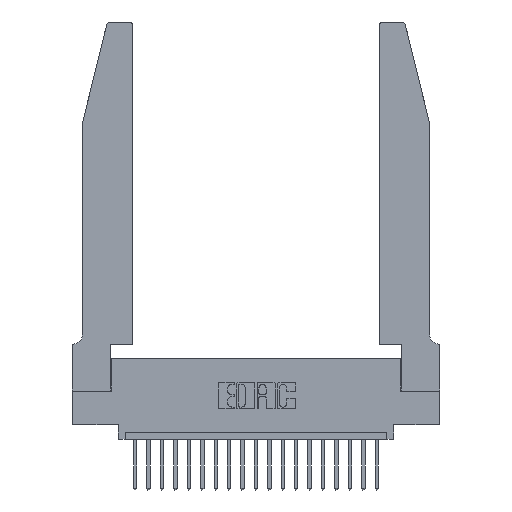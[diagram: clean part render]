
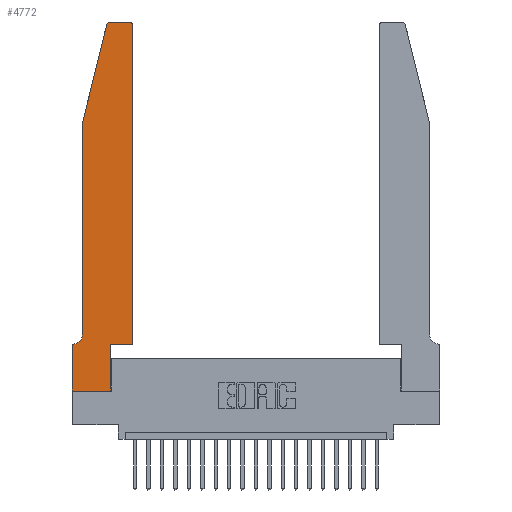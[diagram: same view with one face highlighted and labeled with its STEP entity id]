
A CAD part, top view. The second image highlights one B-rep face of the part: STEP entity #4772.
In plain terms, the highlighted planar face has unit normal (0, 0, 1).
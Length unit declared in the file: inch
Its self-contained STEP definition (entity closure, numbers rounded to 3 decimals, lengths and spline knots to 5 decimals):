
#226 = EDGE_CURVE ( 'NONE', #18353, #14576, #21338, .T. ) ;
#372 = VERTEX_POINT ( 'NONE', #13995 ) ;
#483 = DIRECTION ( 'NONE',  ( 0., 0., 1. ) ) ;
#504 = DIRECTION ( 'NONE',  ( -1., 0., 0. ) ) ;
#871 = VERTEX_POINT ( 'NONE', #3465 ) ;
#1486 = VECTOR ( 'NONE', #11766, 39.37008 ) ;
#1826 = DIRECTION ( 'NONE',  ( 0., -1., 0. ) ) ;
#1968 = ORIENTED_EDGE ( 'NONE', *, *, #3648, .T. ) ;
#2266 = DIRECTION ( 'NONE',  ( 1., 0., 0. ) ) ;
#2371 = EDGE_CURVE ( 'NONE', #14576, #21226, #3385, .T. ) ;
#3284 = DIRECTION ( 'NONE',  ( -1., 0., 0. ) ) ;
#3385 = LINE ( 'NONE', #17024, #1486 ) ;
#3426 = CARTESIAN_POINT ( 'NONE',  ( 0., 0.35, 0.37 ) ) ;
#3465 = CARTESIAN_POINT ( 'NONE',  ( 0.4505, 0.35, 0.37 ) ) ;
#3476 = EDGE_CURVE ( 'NONE', #6200, #7450, #18673, .T. ) ;
#3612 = CIRCLE ( 'NONE', #15629, 0.07 ) ;
#3648 = EDGE_CURVE ( 'NONE', #12119, #12904, #3612, .T. ) ;
#3975 = CARTESIAN_POINT ( 'NONE',  ( 0.0755, 0.42, 0.37 ) ) ;
#4287 = LINE ( 'NONE', #19986, #12368 ) ;
#4311 = VECTOR ( 'NONE', #3284, 39.37008 ) ;
#4448 = VERTEX_POINT ( 'NONE', #13003 ) ;
#4772 = ADVANCED_FACE ( 'NONE', ( #4918 ), #11922, .T. ) ;
#4799 = LINE ( 'NONE', #17687, #5856 ) ;
#4854 = DIRECTION ( 'NONE',  ( 0., 1., 0. ) ) ;
#4918 = FACE_OUTER_BOUND ( 'NONE', #9921, .T. ) ;
#4961 = EDGE_CURVE ( 'NONE', #871, #17091, #15904, .T. ) ;
#5109 = DIRECTION ( 'NONE',  ( 1., 0., 0. ) ) ;
#5128 = ORIENTED_EDGE ( 'NONE', *, *, #3476, .T. ) ;
#5356 = VECTOR ( 'NONE', #1826, 39.37008 ) ;
#5388 = ORIENTED_EDGE ( 'NONE', *, *, #16387, .T. ) ;
#5488 = VERTEX_POINT ( 'NONE', #15908 ) ;
#5856 = VECTOR ( 'NONE', #2266, 39.37008 ) ;
#6200 = VERTEX_POINT ( 'NONE', #21946 ) ;
#6231 = DIRECTION ( 'NONE',  ( -0.239, -0.971, 0. ) ) ;
#6985 = CARTESIAN_POINT ( 'NONE',  ( 0., 0.35, 0.37 ) ) ;
#7149 = EDGE_CURVE ( 'NONE', #5488, #871, #4799, .T. ) ;
#7450 = VERTEX_POINT ( 'NONE', #21586 ) ;
#7591 = CARTESIAN_POINT ( 'NONE',  ( 0.4505, 2.72, 0.37 ) ) ;
#7922 = DIRECTION ( 'NONE',  ( -1., 0., 0. ) ) ;
#7968 = ORIENTED_EDGE ( 'NONE', *, *, #16881, .T. ) ;
#8550 = CARTESIAN_POINT ( 'NONE',  ( 0.2865, 0., 0.37 ) ) ;
#8555 = ORIENTED_EDGE ( 'NONE', *, *, #2371, .T. ) ;
#9391 = CIRCLE ( 'NONE', #11847, 0.03 ) ;
#9405 = CARTESIAN_POINT ( 'NONE',  ( 0.284, 2.72, 0.37 ) ) ;
#9911 = LINE ( 'NONE', #15490, #5356 ) ;
#9921 = EDGE_LOOP ( 'NONE', ( #20059, #5128, #11602, #5388, #1968, #11063, #19698, #8555, #7968, #22237, #12477, #11387 ) ) ;
#10748 = CARTESIAN_POINT ( 'NONE',  ( 0.0055, 0.42, 0.37 ) ) ;
#10884 = EDGE_CURVE ( 'NONE', #17091, #4448, #9391, .T. ) ;
#10956 = LINE ( 'NONE', #11577, #11226 ) ;
#11063 = ORIENTED_EDGE ( 'NONE', *, *, #12961, .T. ) ;
#11213 = DIRECTION ( 'NONE',  ( 0., 0., 1. ) ) ;
#11226 = VECTOR ( 'NONE', #4854, 39.37008 ) ;
#11387 = ORIENTED_EDGE ( 'NONE', *, *, #10884, .T. ) ;
#11577 = CARTESIAN_POINT ( 'NONE',  ( 0.2865, 0.35, 0.37 ) ) ;
#11602 = ORIENTED_EDGE ( 'NONE', *, *, #15414, .T. ) ;
#11766 = DIRECTION ( 'NONE',  ( 1., 0., 0. ) ) ;
#11790 = DIRECTION ( 'NONE',  ( 0., 1., 0. ) ) ;
#11847 = AXIS2_PLACEMENT_3D ( 'NONE', #19638, #483, #17927 ) ;
#11922 = PLANE ( 'NONE',  #14050 ) ;
#12119 = VERTEX_POINT ( 'NONE', #3975 ) ;
#12180 = CARTESIAN_POINT ( 'NONE',  ( 0., 0., 0.37 ) ) ;
#12368 = VECTOR ( 'NONE', #6231, 39.37008 ) ;
#12452 = DIRECTION ( 'NONE',  ( 0., 0., -1. ) ) ;
#12477 = ORIENTED_EDGE ( 'NONE', *, *, #4961, .T. ) ;
#12904 = VERTEX_POINT ( 'NONE', #21538 ) ;
#12961 = EDGE_CURVE ( 'NONE', #12904, #18353, #18152, .T. ) ;
#13003 = CARTESIAN_POINT ( 'NONE',  ( 0.4205, 2.75, 0.37 ) ) ;
#13785 = CARTESIAN_POINT ( 'NONE',  ( 0.2605, 2.75, 0.37 ) ) ;
#13995 = CARTESIAN_POINT ( 'NONE',  ( 0.0755, 2., 0.37 ) ) ;
#14050 = AXIS2_PLACEMENT_3D ( 'NONE', #6985, #15344, #5109 ) ;
#14576 = VERTEX_POINT ( 'NONE', #20952 ) ;
#15344 = DIRECTION ( 'NONE',  ( 0., 0., 1. ) ) ;
#15361 = VECTOR ( 'NONE', #17376, 39.37008 ) ;
#15414 = EDGE_CURVE ( 'NONE', #7450, #372, #4287, .T. ) ;
#15490 = CARTESIAN_POINT ( 'NONE',  ( 0.0755, 2., 0.37 ) ) ;
#15629 = AXIS2_PLACEMENT_3D ( 'NONE', #10748, #12452, #504 ) ;
#15758 = EDGE_CURVE ( 'NONE', #4448, #6200, #17718, .T. ) ;
#15904 = LINE ( 'NONE', #20380, #17793 ) ;
#15908 = CARTESIAN_POINT ( 'NONE',  ( 0.2865, 0.35, 0.37 ) ) ;
#16387 = EDGE_CURVE ( 'NONE', #372, #12119, #9911, .T. ) ;
#16881 = EDGE_CURVE ( 'NONE', #21226, #5488, #10956, .T. ) ;
#17024 = CARTESIAN_POINT ( 'NONE',  ( 0., 0., 0.37 ) ) ;
#17091 = VERTEX_POINT ( 'NONE', #7591 ) ;
#17376 = DIRECTION ( 'NONE',  ( 0., -1., 0. ) ) ;
#17687 = CARTESIAN_POINT ( 'NONE',  ( 0.4505, 0.35, 0.37 ) ) ;
#17718 = LINE ( 'NONE', #13785, #4311 ) ;
#17793 = VECTOR ( 'NONE', #11790, 39.37008 ) ;
#17927 = DIRECTION ( 'NONE',  ( 1., 0., 0. ) ) ;
#17959 = AXIS2_PLACEMENT_3D ( 'NONE', #9405, #11213, #21609 ) ;
#18152 = LINE ( 'NONE', #21755, #19767 ) ;
#18353 = VERTEX_POINT ( 'NONE', #3426 ) ;
#18673 = CIRCLE ( 'NONE', #17959, 0.03 ) ;
#19638 = CARTESIAN_POINT ( 'NONE',  ( 0.4205, 2.72, 0.37 ) ) ;
#19698 = ORIENTED_EDGE ( 'NONE', *, *, #226, .T. ) ;
#19767 = VECTOR ( 'NONE', #7922, 39.37008 ) ;
#19986 = CARTESIAN_POINT ( 'NONE',  ( 0.0755, 2., 0.37 ) ) ;
#20059 = ORIENTED_EDGE ( 'NONE', *, *, #15758, .T. ) ;
#20380 = CARTESIAN_POINT ( 'NONE',  ( 0.4505, 0.35, 0.37 ) ) ;
#20952 = CARTESIAN_POINT ( 'NONE',  ( 0., 0., 0.37 ) ) ;
#21226 = VERTEX_POINT ( 'NONE', #8550 ) ;
#21338 = LINE ( 'NONE', #12180, #15361 ) ;
#21538 = CARTESIAN_POINT ( 'NONE',  ( 0.0055, 0.35, 0.37 ) ) ;
#21586 = CARTESIAN_POINT ( 'NONE',  ( 0.25487, 2.72718, 0.37 ) ) ;
#21609 = DIRECTION ( 'NONE',  ( 1., 0., 0. ) ) ;
#21755 = CARTESIAN_POINT ( 'NONE',  ( 0.0755, 0.35, 0.37 ) ) ;
#21946 = CARTESIAN_POINT ( 'NONE',  ( 0.284, 2.75, 0.37 ) ) ;
#22237 = ORIENTED_EDGE ( 'NONE', *, *, #7149, .T. ) ;
